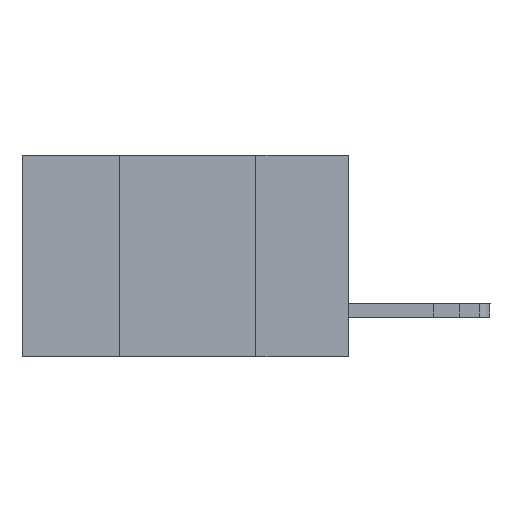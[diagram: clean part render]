
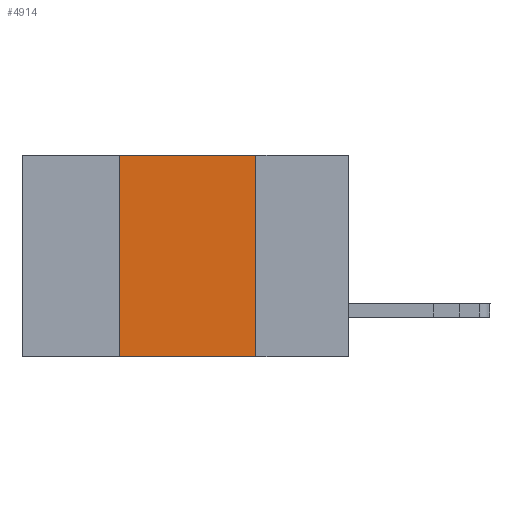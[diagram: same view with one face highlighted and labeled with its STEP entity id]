
A CAD part, left-side view. The second image highlights one B-rep face of the part: STEP entity #4914.
In plain terms, the highlighted planar face has unit normal (-1, 0, 0).
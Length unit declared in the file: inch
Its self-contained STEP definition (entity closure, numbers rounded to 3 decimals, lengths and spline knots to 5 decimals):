
#161 = VERTEX_POINT ( 'NONE', #725 ) ;
#686 = CARTESIAN_POINT ( 'NONE',  ( 0., 0.42, -0.37 ) ) ;
#725 = CARTESIAN_POINT ( 'NONE',  ( 0., 0.17, 0. ) ) ;
#910 = ORIENTED_EDGE ( 'NONE', *, *, #1799, .F. ) ;
#1609 = PLANE ( 'NONE',  #6831 ) ;
#1799 = EDGE_CURVE ( 'NONE', #3714, #161, #2602, .T. ) ;
#2149 = CARTESIAN_POINT ( 'NONE',  ( 0., 0.17, -0.37 ) ) ;
#2355 = CARTESIAN_POINT ( 'NONE',  ( 0., 0.6, 0. ) ) ;
#2602 = LINE ( 'NONE', #7285, #8529 ) ;
#2903 = DIRECTION ( 'NONE',  ( 0., 0., 1. ) ) ;
#3088 = CARTESIAN_POINT ( 'NONE',  ( 0., 0.42, 0. ) ) ;
#3228 = ORIENTED_EDGE ( 'NONE', *, *, #5745, .F. ) ;
#3669 = FACE_OUTER_BOUND ( 'NONE', #5227, .T. ) ;
#3714 = VERTEX_POINT ( 'NONE', #3088 ) ;
#4064 = VERTEX_POINT ( 'NONE', #4599 ) ;
#4166 = CARTESIAN_POINT ( 'NONE',  ( 0., 0.17, -0.37 ) ) ;
#4284 = CARTESIAN_POINT ( 'NONE',  ( 0., 0.6, -0.37 ) ) ;
#4599 = CARTESIAN_POINT ( 'NONE',  ( 0., 0.42, -0.37 ) ) ;
#4658 = DIRECTION ( 'NONE',  ( 1., 0., 0. ) ) ;
#4914 = ADVANCED_FACE ( 'NONE', ( #3669 ), #1609, .F. ) ;
#4974 = DIRECTION ( 'NONE',  ( 0., 0., -1. ) ) ;
#5144 = VECTOR ( 'NONE', #8815, 39.37008 ) ;
#5227 = EDGE_LOOP ( 'NONE', ( #7143, #910, #3228, #8023 ) ) ;
#5240 = VERTEX_POINT ( 'NONE', #2149 ) ;
#5644 = DIRECTION ( 'NONE',  ( 0., -1., 0. ) ) ;
#5745 = EDGE_CURVE ( 'NONE', #4064, #3714, #6827, .T. ) ;
#6827 = LINE ( 'NONE', #686, #7493 ) ;
#6831 = AXIS2_PLACEMENT_3D ( 'NONE', #2355, #4658, #9088 ) ;
#7128 = LINE ( 'NONE', #4284, #5144 ) ;
#7143 = ORIENTED_EDGE ( 'NONE', *, *, #7772, .F. ) ;
#7285 = CARTESIAN_POINT ( 'NONE',  ( 0., 0.6, 0. ) ) ;
#7493 = VECTOR ( 'NONE', #2903, 39.37008 ) ;
#7772 = EDGE_CURVE ( 'NONE', #161, #5240, #8746, .T. ) ;
#8023 = ORIENTED_EDGE ( 'NONE', *, *, #8412, .T. ) ;
#8412 = EDGE_CURVE ( 'NONE', #4064, #5240, #7128, .T. ) ;
#8462 = VECTOR ( 'NONE', #4974, 39.37008 ) ;
#8529 = VECTOR ( 'NONE', #5644, 39.37008 ) ;
#8746 = LINE ( 'NONE', #4166, #8462 ) ;
#8815 = DIRECTION ( 'NONE',  ( 0., -1., 0. ) ) ;
#9088 = DIRECTION ( 'NONE',  ( 0., 0., -1. ) ) ;
